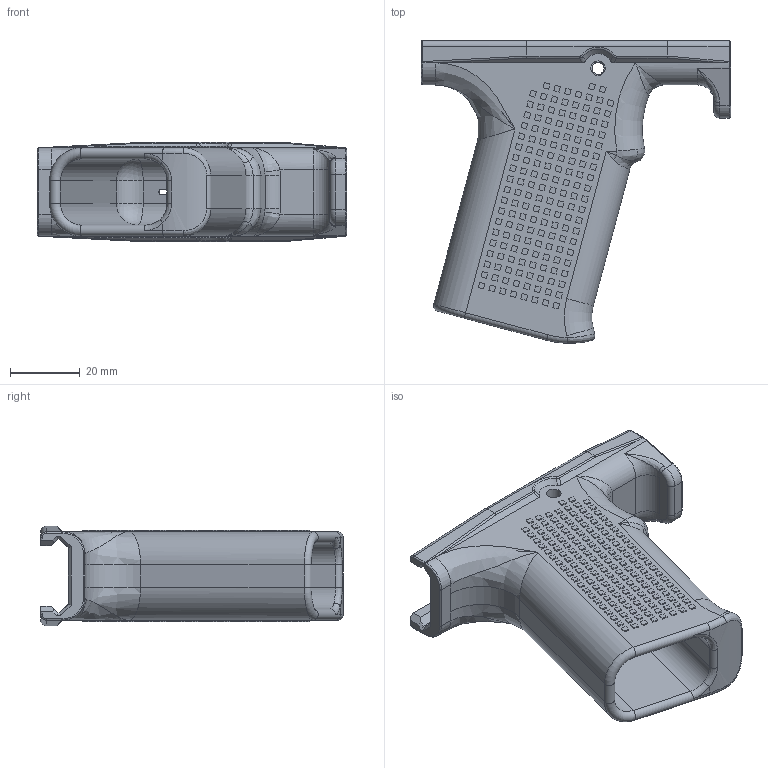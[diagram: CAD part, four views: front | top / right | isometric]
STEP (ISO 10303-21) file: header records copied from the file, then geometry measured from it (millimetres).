
FILE_DESCRIPTION(/* description */ (''),/* implementation_level */ '2;1');
FILE_NAME(/* name */ 'G34FG.stp',/* time_stamp */ '2018-09-10T19:30:57-04:00',/* author */ ('Admin'),/* organization */ (''),/* preprocessor_version */ 'ST-DEVELOPER v16.1',/* originating_system */ 'Autodesk Inventor 2016',/* authorisation */ '');
FILE_SCHEMA (('AUTOMOTIVE_DESIGN { 1 0 10303 214 3 1 1 }'));
Length unit declared in the file: inch
Products named in the file (1): G34FG
Bounding box: 88.9 x 87 x 28.57 mm (x, y, z)
Volume: 57232.3 mm3; surface area: 25330.9 mm2
Topology: 1 solids, 1 shells, 1813 faces, 4365 edges, 2864 vertices
Faces by surface type: plane 1674, cylinder 71, bspline 40, torus 22, sphere 4, cone 2
Full cylindrical faces by diameter (mm): 3.454 x1, 4.216 x1
Entity records: 52910 total; most frequent: CARTESIAN_POINT 10612, ORIENTED_EDGE 8710, DIRECTION 8021, EDGE_CURVE 4355, LINE 4097, VECTOR 4097, VERTEX_POINT 2864, EDGE_LOOP 2139
